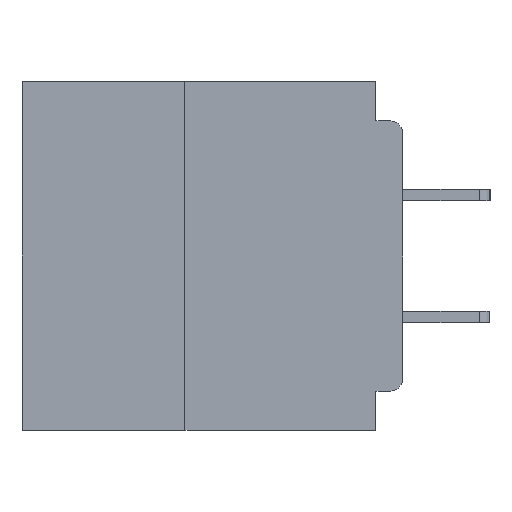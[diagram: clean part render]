
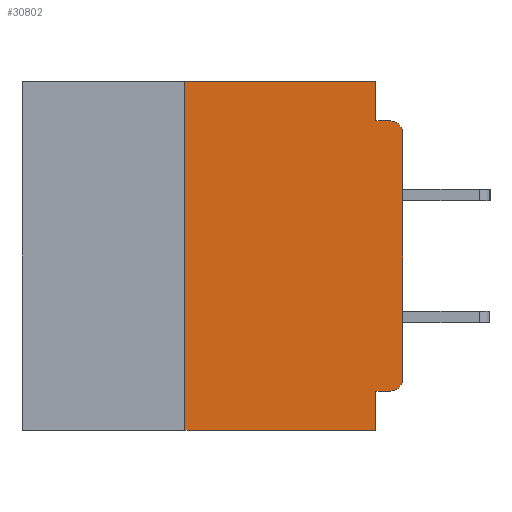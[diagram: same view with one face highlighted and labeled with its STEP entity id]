
A CAD part, left-side view. The second image highlights one B-rep face of the part: STEP entity #30802.
In plain terms, the highlighted planar face has unit normal (-1, 0, 0).
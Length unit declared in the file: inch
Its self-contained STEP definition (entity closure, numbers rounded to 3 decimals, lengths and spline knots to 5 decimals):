
#304 = DIRECTION ( 'NONE',  ( 0., -1., 0. ) ) ;
#1621 = CIRCLE ( 'NONE', #20618, 0.015 ) ;
#2326 = ORIENTED_EDGE ( 'NONE', *, *, #24563, .T. ) ;
#2344 = CARTESIAN_POINT ( 'NONE',  ( 0., 0.015, -0.045 ) ) ;
#2420 = EDGE_CURVE ( 'NONE', #53993, #46403, #7515, .T. ) ;
#2968 = VECTOR ( 'NONE', #19505, 39.37008 ) ;
#3448 = EDGE_CURVE ( 'NONE', #19957, #11363, #25702, .T. ) ;
#3922 = AXIS2_PLACEMENT_3D ( 'NONE', #15410, #62967, #31471 ) ;
#3934 = CARTESIAN_POINT ( 'NONE',  ( 0., 0.031, -0.045 ) ) ;
#4091 = DIRECTION ( 'NONE',  ( 0., 0., 1. ) ) ;
#4334 = CARTESIAN_POINT ( 'NONE',  ( 0., 0.031, 0. ) ) ;
#4438 = CARTESIAN_POINT ( 'NONE',  ( 0., 0.031, -0.4 ) ) ;
#4499 = VECTOR ( 'NONE', #36265, 39.37008 ) ;
#4906 = EDGE_CURVE ( 'NONE', #19957, #49850, #18788, .T. ) ;
#7515 = LINE ( 'NONE', #60802, #63750 ) ;
#8706 = DIRECTION ( 'NONE',  ( 0., -1., 0. ) ) ;
#9286 = EDGE_CURVE ( 'NONE', #49850, #59742, #30133, .T. ) ;
#9352 = ORIENTED_EDGE ( 'NONE', *, *, #21745, .F. ) ;
#11029 = VERTEX_POINT ( 'NONE', #3934 ) ;
#11276 = CARTESIAN_POINT ( 'NONE',  ( 0., 0.25, 0. ) ) ;
#11363 = VERTEX_POINT ( 'NONE', #43760 ) ;
#12426 = ORIENTED_EDGE ( 'NONE', *, *, #54745, .F. ) ;
#12572 = VERTEX_POINT ( 'NONE', #2344 ) ;
#14317 = CARTESIAN_POINT ( 'NONE',  ( 0., 0.015, -0.06 ) ) ;
#14626 = CARTESIAN_POINT ( 'NONE',  ( 0., 0.015, -0.34 ) ) ;
#15410 = CARTESIAN_POINT ( 'NONE',  ( 0., 0.437, 0. ) ) ;
#18529 = ORIENTED_EDGE ( 'NONE', *, *, #3448, .T. ) ;
#18647 = LINE ( 'NONE', #4438, #4499 ) ;
#18788 = LINE ( 'NONE', #19032, #2968 ) ;
#19032 = CARTESIAN_POINT ( 'NONE',  ( 0., 0.25, -0.4 ) ) ;
#19505 = DIRECTION ( 'NONE',  ( 0., 0., 1. ) ) ;
#19650 = DIRECTION ( 'NONE',  ( 0., 0., -1. ) ) ;
#19957 = VERTEX_POINT ( 'NONE', #43886 ) ;
#19961 = DIRECTION ( 'NONE',  ( 0., 0., -1. ) ) ;
#20618 = AXIS2_PLACEMENT_3D ( 'NONE', #14626, #51559, #19961 ) ;
#21745 = EDGE_CURVE ( 'NONE', #11029, #12572, #47522, .T. ) ;
#23036 = VECTOR ( 'NONE', #51984, 39.37008 ) ;
#23232 = LINE ( 'NONE', #57038, #63601 ) ;
#23976 = EDGE_CURVE ( 'NONE', #53993, #54393, #1621, .T. ) ;
#24497 = DIRECTION ( 'NONE',  ( 0., -1., 0. ) ) ;
#24539 = CARTESIAN_POINT ( 'NONE',  ( 0., 0.437, 0. ) ) ;
#24563 = EDGE_CURVE ( 'NONE', #54393, #66157, #23232, .T. ) ;
#25186 = ORIENTED_EDGE ( 'NONE', *, *, #9286, .F. ) ;
#25702 = LINE ( 'NONE', #26489, #38102 ) ;
#26129 = PLANE ( 'NONE',  #3922 ) ;
#26489 = CARTESIAN_POINT ( 'NONE',  ( 0., 0.437, -0.4 ) ) ;
#30133 = LINE ( 'NONE', #24539, #42471 ) ;
#30679 = ORIENTED_EDGE ( 'NONE', *, *, #4906, .F. ) ;
#30802 = ADVANCED_FACE ( 'NONE', ( #61101 ), #26129, .F. ) ;
#31471 = DIRECTION ( 'NONE',  ( 0., 0., -1. ) ) ;
#33411 = CARTESIAN_POINT ( 'NONE',  ( 0., 0.015, -0.355 ) ) ;
#35727 = CARTESIAN_POINT ( 'NONE',  ( 0., 0.031, -0.355 ) ) ;
#36265 = DIRECTION ( 'NONE',  ( 0., 0., -1. ) ) ;
#36306 = CARTESIAN_POINT ( 'NONE',  ( 0., 0.031, 0. ) ) ;
#36977 = AXIS2_PLACEMENT_3D ( 'NONE', #14317, #51248, #19650 ) ;
#37269 = ORIENTED_EDGE ( 'NONE', *, *, #23976, .T. ) ;
#37455 = CARTESIAN_POINT ( 'NONE',  ( 0., 0., -0.045 ) ) ;
#38102 = VECTOR ( 'NONE', #24497, 39.37008 ) ;
#42471 = VECTOR ( 'NONE', #8706, 39.37008 ) ;
#42681 = EDGE_CURVE ( 'NONE', #66157, #12572, #67995, .T. ) ;
#43760 = CARTESIAN_POINT ( 'NONE',  ( 0., 0.031, -0.4 ) ) ;
#43886 = CARTESIAN_POINT ( 'NONE',  ( 0., 0.25, -0.4 ) ) ;
#44226 = ORIENTED_EDGE ( 'NONE', *, *, #42681, .T. ) ;
#46403 = VERTEX_POINT ( 'NONE', #35727 ) ;
#47522 = LINE ( 'NONE', #37455, #59860 ) ;
#47982 = ORIENTED_EDGE ( 'NONE', *, *, #2420, .F. ) ;
#49413 = EDGE_LOOP ( 'NONE', ( #2326, #44226, #9352, #12426, #25186, #30679, #18529, #66486, #47982, #37269 ) ) ;
#49850 = VERTEX_POINT ( 'NONE', #11276 ) ;
#51248 = DIRECTION ( 'NONE',  ( -1., 0., 0. ) ) ;
#51559 = DIRECTION ( 'NONE',  ( -1., 0., 0. ) ) ;
#51984 = DIRECTION ( 'NONE',  ( 0., 0., -1. ) ) ;
#53993 = VERTEX_POINT ( 'NONE', #33411 ) ;
#54393 = VERTEX_POINT ( 'NONE', #58658 ) ;
#54745 = EDGE_CURVE ( 'NONE', #59742, #11029, #65057, .T. ) ;
#55929 = EDGE_CURVE ( 'NONE', #46403, #11363, #18647, .T. ) ;
#57038 = CARTESIAN_POINT ( 'NONE',  ( 0., 0., 0. ) ) ;
#58658 = CARTESIAN_POINT ( 'NONE',  ( 0., 0., -0.34 ) ) ;
#59742 = VERTEX_POINT ( 'NONE', #36306 ) ;
#59860 = VECTOR ( 'NONE', #304, 39.37008 ) ;
#60802 = CARTESIAN_POINT ( 'NONE',  ( 0., 0., -0.355 ) ) ;
#61031 = DIRECTION ( 'NONE',  ( 0., 1., 0. ) ) ;
#61101 = FACE_OUTER_BOUND ( 'NONE', #49413, .T. ) ;
#62967 = DIRECTION ( 'NONE',  ( 1., 0., 0. ) ) ;
#63601 = VECTOR ( 'NONE', #4091, 39.37008 ) ;
#63750 = VECTOR ( 'NONE', #61031, 39.37008 ) ;
#65057 = LINE ( 'NONE', #4334, #23036 ) ;
#65617 = CARTESIAN_POINT ( 'NONE',  ( 0., 0., -0.06 ) ) ;
#66157 = VERTEX_POINT ( 'NONE', #65617 ) ;
#66486 = ORIENTED_EDGE ( 'NONE', *, *, #55929, .F. ) ;
#67995 = CIRCLE ( 'NONE', #36977, 0.015 ) ;
